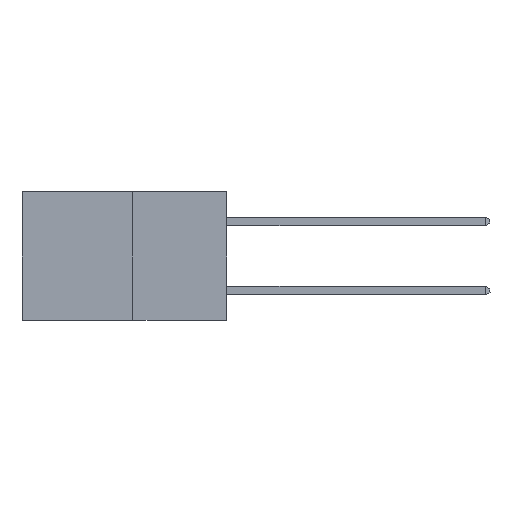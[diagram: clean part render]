
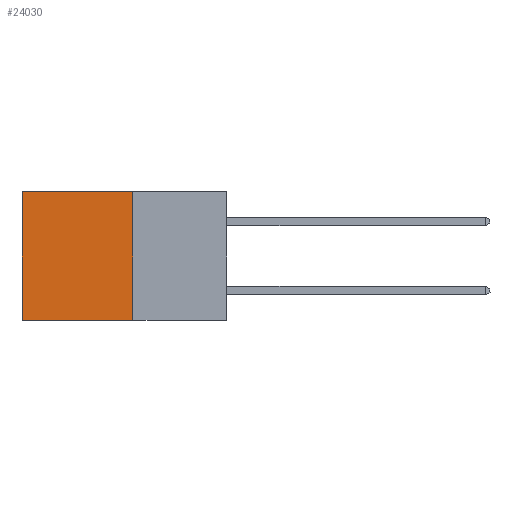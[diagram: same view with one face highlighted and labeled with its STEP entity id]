
A CAD part, left-side view. The second image highlights one B-rep face of the part: STEP entity #24030.
In plain terms, the highlighted planar face has unit normal (-1, 0, 0).
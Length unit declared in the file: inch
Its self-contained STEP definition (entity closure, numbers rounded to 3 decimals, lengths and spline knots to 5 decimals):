
#189 = CARTESIAN_POINT ( 'NONE',  ( 0.277, 0.59, 0. ) ) ;
#767 = CARTESIAN_POINT ( 'NONE',  ( 0.277, 0.27, 0. ) ) ;
#872 = EDGE_CURVE ( 'NONE', #20425, #8258, #20653, .T. ) ;
#1040 = CARTESIAN_POINT ( 'NONE',  ( 0.277, 0.27, -0.37 ) ) ;
#1986 = VECTOR ( 'NONE', #14376, 39.37008 ) ;
#4323 = CARTESIAN_POINT ( 'NONE',  ( 0.277, 0.27, -0.37 ) ) ;
#4593 = LINE ( 'NONE', #12949, #15594 ) ;
#7751 = DIRECTION ( 'NONE',  ( 0., 0., -1. ) ) ;
#8258 = VERTEX_POINT ( 'NONE', #189 ) ;
#9308 = VECTOR ( 'NONE', #17478, 39.37008 ) ;
#9882 = ORIENTED_EDGE ( 'NONE', *, *, #26274, .T. ) ;
#9900 = ORIENTED_EDGE ( 'NONE', *, *, #11034, .F. ) ;
#11034 = EDGE_CURVE ( 'NONE', #20425, #12869, #20244, .T. ) ;
#11079 = CARTESIAN_POINT ( 'NONE',  ( 0.277, 0.27, 0. ) ) ;
#12152 = ORIENTED_EDGE ( 'NONE', *, *, #24051, .F. ) ;
#12205 = CARTESIAN_POINT ( 'NONE',  ( 0.277, 0.27, -0.37 ) ) ;
#12869 = VERTEX_POINT ( 'NONE', #18022 ) ;
#12949 = CARTESIAN_POINT ( 'NONE',  ( 0.277, 0.59, -0.37 ) ) ;
#13769 = LINE ( 'NONE', #12205, #1986 ) ;
#14154 = VECTOR ( 'NONE', #14928, 39.37008 ) ;
#14376 = DIRECTION ( 'NONE',  ( 0., 1., 0. ) ) ;
#14928 = DIRECTION ( 'NONE',  ( 0., 1., 0. ) ) ;
#15594 = VECTOR ( 'NONE', #19526, 39.37008 ) ;
#17478 = DIRECTION ( 'NONE',  ( 0., 0., -1. ) ) ;
#18022 = CARTESIAN_POINT ( 'NONE',  ( 0.277, 0.27, -0.37 ) ) ;
#19526 = DIRECTION ( 'NONE',  ( 0., 0., -1. ) ) ;
#20244 = LINE ( 'NONE', #4323, #9308 ) ;
#20425 = VERTEX_POINT ( 'NONE', #767 ) ;
#20653 = LINE ( 'NONE', #11079, #14154 ) ;
#20861 = DIRECTION ( 'NONE',  ( 1., 0., 0. ) ) ;
#21542 = ORIENTED_EDGE ( 'NONE', *, *, #872, .T. ) ;
#21652 = CARTESIAN_POINT ( 'NONE',  ( 0.277, 0.59, -0.37 ) ) ;
#21936 = EDGE_LOOP ( 'NONE', ( #9882, #12152, #9900, #21542 ) ) ;
#22942 = PLANE ( 'NONE',  #23375 ) ;
#23375 = AXIS2_PLACEMENT_3D ( 'NONE', #1040, #20861, #7751 ) ;
#24030 = ADVANCED_FACE ( 'NONE', ( #25281 ), #22942, .F. ) ;
#24051 = EDGE_CURVE ( 'NONE', #12869, #26853, #13769, .T. ) ;
#25281 = FACE_OUTER_BOUND ( 'NONE', #21936, .T. ) ;
#26274 = EDGE_CURVE ( 'NONE', #8258, #26853, #4593, .T. ) ;
#26853 = VERTEX_POINT ( 'NONE', #21652 ) ;
